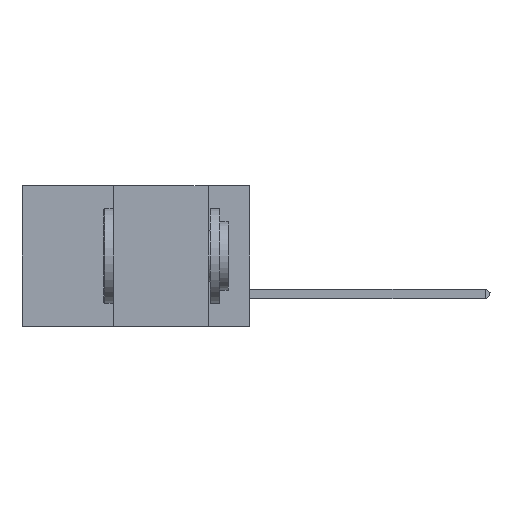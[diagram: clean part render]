
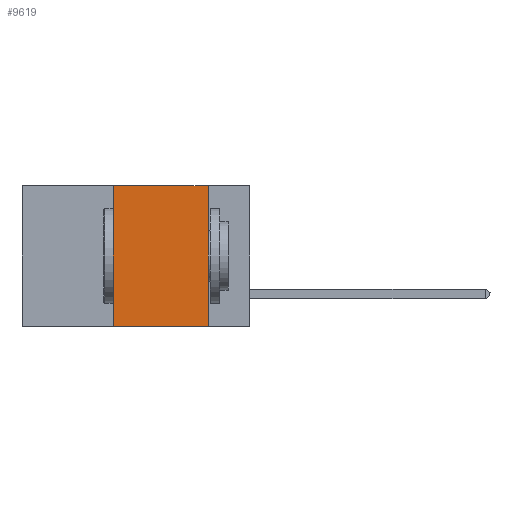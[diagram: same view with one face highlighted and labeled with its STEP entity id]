
A CAD part, left-side view. The second image highlights one B-rep face of the part: STEP entity #9619.
In plain terms, the highlighted planar face has unit normal (-1, 0, 0).
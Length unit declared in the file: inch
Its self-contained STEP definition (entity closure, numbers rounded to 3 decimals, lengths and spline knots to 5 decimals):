
#173 = DIRECTION ( 'NONE',  ( 0., 0., 1. ) ) ;
#1066 = LINE ( 'NONE', #34120, #36756 ) ;
#1096 = AXIS2_PLACEMENT_3D ( 'NONE', #24102, #5168, #4337 ) ;
#2354 = ORIENTED_EDGE ( 'NONE', *, *, #26588, .F. ) ;
#3113 = CARTESIAN_POINT ( 'NONE',  ( 0., 0.11, 0. ) ) ;
#4337 = DIRECTION ( 'NONE',  ( 0., 0., -1. ) ) ;
#4535 = EDGE_CURVE ( 'NONE', #35050, #9883, #13579, .T. ) ;
#5168 = DIRECTION ( 'NONE',  ( 1., 0., 0. ) ) ;
#5814 = EDGE_CURVE ( 'NONE', #9883, #39903, #27618, .T. ) ;
#5894 = DIRECTION ( 'NONE',  ( 0., -1., 0. ) ) ;
#6194 = CARTESIAN_POINT ( 'NONE',  ( 0., 0.11, -0.37 ) ) ;
#6584 = FACE_OUTER_BOUND ( 'NONE', #40665, .T. ) ;
#7416 = CARTESIAN_POINT ( 'NONE',  ( 0., 0.36, -0.37 ) ) ;
#8808 = LINE ( 'NONE', #3113, #14711 ) ;
#9619 = ADVANCED_FACE ( 'NONE', ( #6584 ), #11545, .F. ) ;
#9883 = VERTEX_POINT ( 'NONE', #12483 ) ;
#11545 = PLANE ( 'NONE',  #1096 ) ;
#12483 = CARTESIAN_POINT ( 'NONE',  ( 0., 0.36, 0. ) ) ;
#12606 = VECTOR ( 'NONE', #173, 39.37008 ) ;
#12693 = EDGE_CURVE ( 'NONE', #35050, #20806, #1066, .T. ) ;
#13579 = LINE ( 'NONE', #25110, #12606 ) ;
#14711 = VECTOR ( 'NONE', #31630, 39.37008 ) ;
#15729 = ORIENTED_EDGE ( 'NONE', *, *, #5814, .F. ) ;
#17082 = ORIENTED_EDGE ( 'NONE', *, *, #12693, .T. ) ;
#19668 = VECTOR ( 'NONE', #30799, 39.37008 ) ;
#20806 = VERTEX_POINT ( 'NONE', #6194 ) ;
#21247 = CARTESIAN_POINT ( 'NONE',  ( 0., 0.11, 0. ) ) ;
#24102 = CARTESIAN_POINT ( 'NONE',  ( 0., 0.6, 0. ) ) ;
#25110 = CARTESIAN_POINT ( 'NONE',  ( 0., 0.36, 0. ) ) ;
#26327 = ORIENTED_EDGE ( 'NONE', *, *, #4535, .F. ) ;
#26588 = EDGE_CURVE ( 'NONE', #39903, #20806, #8808, .T. ) ;
#27618 = LINE ( 'NONE', #31349, #19668 ) ;
#30799 = DIRECTION ( 'NONE',  ( 0., -1., 0. ) ) ;
#31349 = CARTESIAN_POINT ( 'NONE',  ( 0., 0.6, 0. ) ) ;
#31630 = DIRECTION ( 'NONE',  ( 0., 0., -1. ) ) ;
#34120 = CARTESIAN_POINT ( 'NONE',  ( 0., 0.6, -0.37 ) ) ;
#35050 = VERTEX_POINT ( 'NONE', #7416 ) ;
#36756 = VECTOR ( 'NONE', #5894, 39.37008 ) ;
#39903 = VERTEX_POINT ( 'NONE', #21247 ) ;
#40665 = EDGE_LOOP ( 'NONE', ( #2354, #15729, #26327, #17082 ) ) ;
